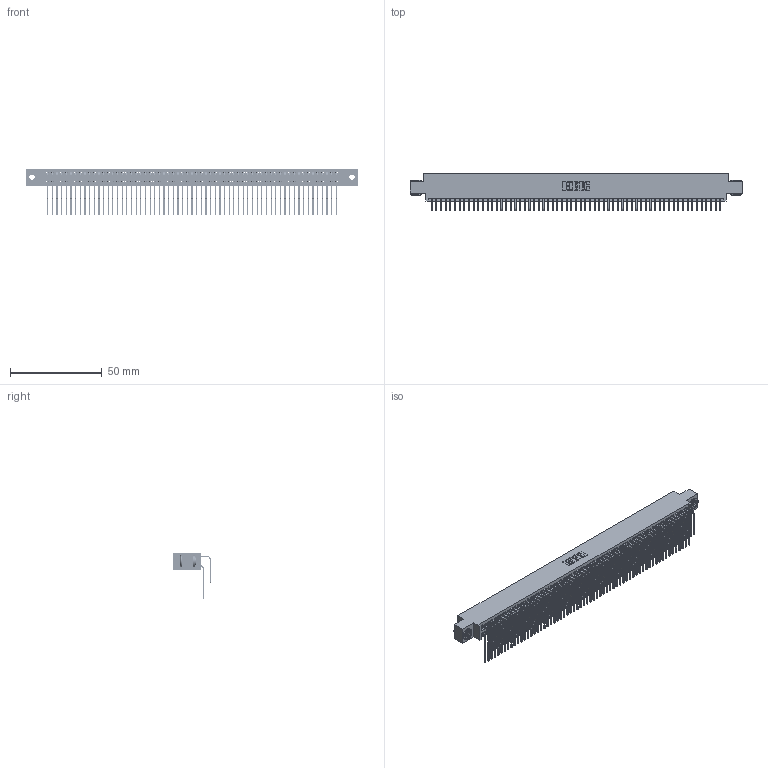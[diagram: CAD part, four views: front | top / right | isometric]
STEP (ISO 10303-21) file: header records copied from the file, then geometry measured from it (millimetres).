
FILE_DESCRIPTION (( 'STEP AP203' ), '1' );
FILE_NAME ('395-126-559-803.STEP', '2019-10-28T17:07:05', ( '' ), ( '' ), 'SwSTEP 2.0', 'SolidWorks 2016', '' );
FILE_SCHEMA (( 'CONFIG_CONTROL_DESIGN' ));
Length unit declared in the file: inch
Products named in the file (5): 345-292-001_559 Tail - 2; 345-250-002_345-250-002-102; 395-126-559-803; 345-292-001_558 559 Tail - 1; 345 Part_0.170 Offset - 0.156 Dia-TH
Assembly tree (129 placements, depth 2):
  395-126-559-803
    345 Part_0.170 Offset - 0.156 Dia-TH
    345-292-001_558 559 Tail - 1  x63
    345-292-001_559 Tail - 2  x63
    345-250-002_345-250-002-102  x2
Bounding box: 181.23 x 20.56 x 25.53 mm (x, y, z)
Volume: 18432.6 mm3; surface area: 31419.5 mm2
Topology: 129 solids, 129 shells, 6720 faces, 19959 edges, 13134 vertices
Faces by surface type: plane 4504, cylinder 2208, cone 8
Entity records: 49038 total; most frequent: CARTESIAN_POINT 8222, ORIENTED_EDGE 8098, DIRECTION 7227, EDGE_CURVE 4049, LINE 3601, VECTOR 3601, VERTEX_POINT 2694, AXIS2_PLACEMENT_3D 1813
